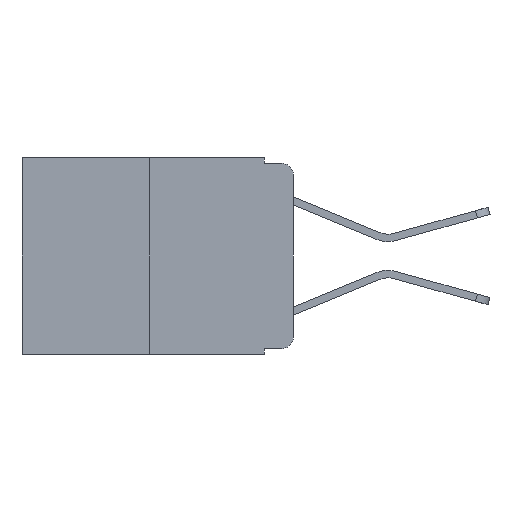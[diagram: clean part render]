
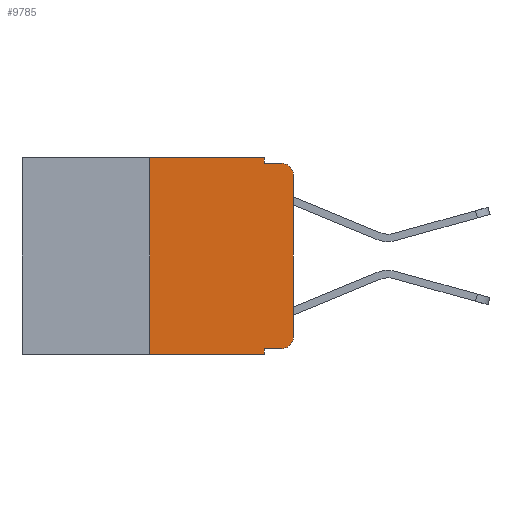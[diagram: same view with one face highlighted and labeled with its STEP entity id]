
A CAD part, left-side view. The second image highlights one B-rep face of the part: STEP entity #9785.
In plain terms, the highlighted planar face has unit normal (-1, 0, 0).
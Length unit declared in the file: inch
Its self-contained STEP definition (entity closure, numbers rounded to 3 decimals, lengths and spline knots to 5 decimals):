
#29 = CARTESIAN_POINT ( 'NONE',  ( 0., 0., -0.03 ) ) ;
#54 = ORIENTED_EDGE ( 'NONE', *, *, #532, .T. ) ;
#312 = DIRECTION ( 'NONE',  ( 0., 0., -1. ) ) ;
#532 = EDGE_CURVE ( 'NONE', #18215, #13617, #2265, .T. ) ;
#755 = ORIENTED_EDGE ( 'NONE', *, *, #18234, .F. ) ;
#1503 = CARTESIAN_POINT ( 'NONE',  ( 0., 0.02, -0.01 ) ) ;
#1587 = ORIENTED_EDGE ( 'NONE', *, *, #15588, .F. ) ;
#1717 = ORIENTED_EDGE ( 'NONE', *, *, #14728, .F. ) ;
#1874 = LINE ( 'NONE', #13675, #6560 ) ;
#2204 = ORIENTED_EDGE ( 'NONE', *, *, #4058, .T. ) ;
#2242 = ORIENTED_EDGE ( 'NONE', *, *, #6500, .T. ) ;
#2265 = LINE ( 'NONE', #9669, #10185 ) ;
#2419 = LINE ( 'NONE', #9902, #7608 ) ;
#2456 = ORIENTED_EDGE ( 'NONE', *, *, #3006, .T. ) ;
#3006 = EDGE_CURVE ( 'NONE', #5510, #13340, #19177, .T. ) ;
#3341 = EDGE_CURVE ( 'NONE', #8167, #13340, #18022, .T. ) ;
#3422 = CARTESIAN_POINT ( 'NONE',  ( 0., 0.02, -0.333 ) ) ;
#3570 = VERTEX_POINT ( 'NONE', #11147 ) ;
#3779 = EDGE_CURVE ( 'NONE', #19478, #7018, #13969, .T. ) ;
#4058 = EDGE_CURVE ( 'NONE', #6140, #5510, #5818, .T. ) ;
#4859 = VECTOR ( 'NONE', #5967, 39.37008 ) ;
#5138 = AXIS2_PLACEMENT_3D ( 'NONE', #6890, #8531, #19231 ) ;
#5378 = DIRECTION ( 'NONE',  ( 0., -1., 0. ) ) ;
#5510 = VERTEX_POINT ( 'NONE', #29 ) ;
#5816 = DIRECTION ( 'NONE',  ( 0., -1., 0. ) ) ;
#5818 = LINE ( 'NONE', #16882, #4859 ) ;
#5967 = DIRECTION ( 'NONE',  ( 0., 0., 1. ) ) ;
#6140 = VERTEX_POINT ( 'NONE', #19869 ) ;
#6272 = CARTESIAN_POINT ( 'NONE',  ( 0., 0.051, 0. ) ) ;
#6277 = AXIS2_PLACEMENT_3D ( 'NONE', #8522, #19220, #10088 ) ;
#6381 = LINE ( 'NONE', #7883, #18272 ) ;
#6500 = EDGE_CURVE ( 'NONE', #7018, #6140, #17479, .T. ) ;
#6560 = VECTOR ( 'NONE', #5816, 39.37008 ) ;
#6712 = CARTESIAN_POINT ( 'NONE',  ( 0., 0.051, -0.333 ) ) ;
#6890 = CARTESIAN_POINT ( 'NONE',  ( 0., 0.473, 0. ) ) ;
#7018 = VERTEX_POINT ( 'NONE', #3422 ) ;
#7408 = CARTESIAN_POINT ( 'NONE',  ( 0., 0.051, -0.01 ) ) ;
#7608 = VECTOR ( 'NONE', #312, 39.37008 ) ;
#7809 = CARTESIAN_POINT ( 'NONE',  ( 0., 0.25, -0.343 ) ) ;
#7883 = CARTESIAN_POINT ( 'NONE',  ( 0., 0.25, 0. ) ) ;
#8097 = CARTESIAN_POINT ( 'NONE',  ( 0., 0.051, -0.01 ) ) ;
#8167 = VERTEX_POINT ( 'NONE', #8097 ) ;
#8295 = ORIENTED_EDGE ( 'NONE', *, *, #3341, .F. ) ;
#8522 = CARTESIAN_POINT ( 'NONE',  ( 0., 0.02, -0.313 ) ) ;
#8531 = DIRECTION ( 'NONE',  ( 1., 0., 0. ) ) ;
#8865 = ORIENTED_EDGE ( 'NONE', *, *, #19907, .F. ) ;
#9020 = DIRECTION ( 'NONE',  ( 0., -1., 0. ) ) ;
#9482 = DIRECTION ( 'NONE',  ( 0., 0., 1. ) ) ;
#9522 = AXIS2_PLACEMENT_3D ( 'NONE', #10824, #16872, #16388 ) ;
#9669 = CARTESIAN_POINT ( 'NONE',  ( 0., 0.473, -0.343 ) ) ;
#9785 = ADVANCED_FACE ( 'NONE', ( #15503 ), #10028, .F. ) ;
#9798 = ORIENTED_EDGE ( 'NONE', *, *, #3779, .T. ) ;
#9902 = CARTESIAN_POINT ( 'NONE',  ( 0., 0.051, 0. ) ) ;
#10028 = PLANE ( 'NONE',  #5138 ) ;
#10065 = LINE ( 'NONE', #6272, #17273 ) ;
#10088 = DIRECTION ( 'NONE',  ( 0., 0., -1. ) ) ;
#10185 = VECTOR ( 'NONE', #16884, 39.37008 ) ;
#10824 = CARTESIAN_POINT ( 'NONE',  ( 0., 0.02, -0.03 ) ) ;
#11147 = CARTESIAN_POINT ( 'NONE',  ( 0., 0.051, 0. ) ) ;
#13339 = CARTESIAN_POINT ( 'NONE',  ( 0., 0.051, -0.343 ) ) ;
#13340 = VERTEX_POINT ( 'NONE', #1503 ) ;
#13617 = VERTEX_POINT ( 'NONE', #13339 ) ;
#13675 = CARTESIAN_POINT ( 'NONE',  ( 0., 0.473, 0. ) ) ;
#13969 = LINE ( 'NONE', #14788, #18003 ) ;
#14728 = EDGE_CURVE ( 'NONE', #19478, #13617, #2419, .T. ) ;
#14788 = CARTESIAN_POINT ( 'NONE',  ( 0., 0.051, -0.333 ) ) ;
#15503 = FACE_OUTER_BOUND ( 'NONE', #19943, .T. ) ;
#15588 = EDGE_CURVE ( 'NONE', #18360, #3570, #1874, .T. ) ;
#15640 = DIRECTION ( 'NONE',  ( 0., 0., -1. ) ) ;
#15935 = CARTESIAN_POINT ( 'NONE',  ( 0., 0.25, 0. ) ) ;
#16388 = DIRECTION ( 'NONE',  ( 0., 0., -1. ) ) ;
#16872 = DIRECTION ( 'NONE',  ( -1., 0., 0. ) ) ;
#16882 = CARTESIAN_POINT ( 'NONE',  ( 0., 0., 0. ) ) ;
#16884 = DIRECTION ( 'NONE',  ( 0., -1., 0. ) ) ;
#17077 = VECTOR ( 'NONE', #9020, 39.37008 ) ;
#17273 = VECTOR ( 'NONE', #15640, 39.37008 ) ;
#17479 = CIRCLE ( 'NONE', #6277, 0.02 ) ;
#18003 = VECTOR ( 'NONE', #5378, 39.37008 ) ;
#18022 = LINE ( 'NONE', #7408, #17077 ) ;
#18215 = VERTEX_POINT ( 'NONE', #7809 ) ;
#18234 = EDGE_CURVE ( 'NONE', #18215, #18360, #6381, .T. ) ;
#18272 = VECTOR ( 'NONE', #9482, 39.37008 ) ;
#18360 = VERTEX_POINT ( 'NONE', #15935 ) ;
#19177 = CIRCLE ( 'NONE', #9522, 0.02 ) ;
#19220 = DIRECTION ( 'NONE',  ( -1., 0., 0. ) ) ;
#19231 = DIRECTION ( 'NONE',  ( 0., 0., -1. ) ) ;
#19478 = VERTEX_POINT ( 'NONE', #6712 ) ;
#19869 = CARTESIAN_POINT ( 'NONE',  ( 0., 0., -0.313 ) ) ;
#19907 = EDGE_CURVE ( 'NONE', #3570, #8167, #10065, .T. ) ;
#19943 = EDGE_LOOP ( 'NONE', ( #2204, #2456, #8295, #8865, #1587, #755, #54, #1717, #9798, #2242 ) ) ;
